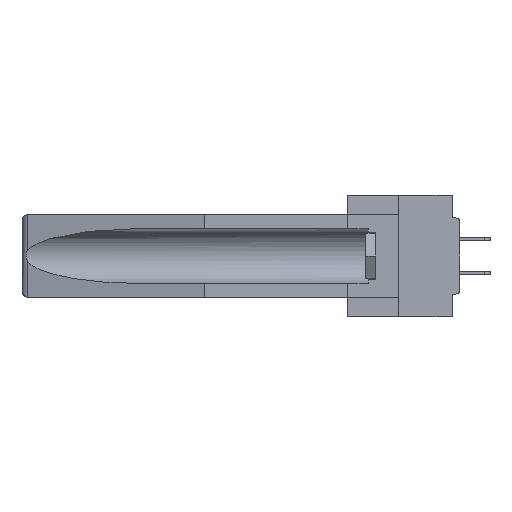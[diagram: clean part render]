
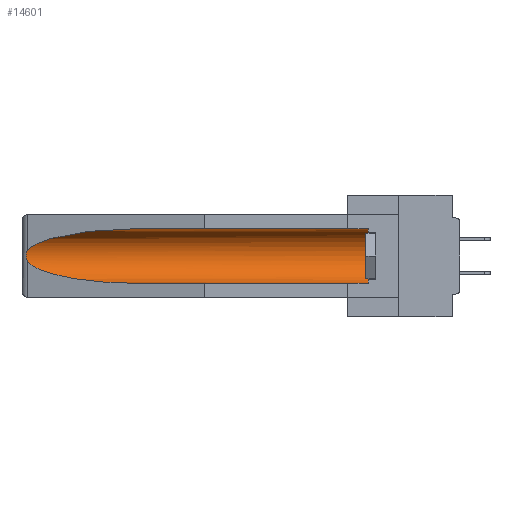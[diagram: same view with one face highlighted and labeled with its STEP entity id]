
A CAD part, left-side view. The second image highlights one B-rep face of the part: STEP entity #14601.
In plain terms, the highlighted cylindrical face has radius 2.857 mm (diameter 5.715 mm), a partial arc.
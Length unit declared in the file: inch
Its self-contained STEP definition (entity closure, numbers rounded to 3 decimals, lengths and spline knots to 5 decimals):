
#1794 = VERTEX_POINT ( 'NONE', #40493 ) ;
#1892 = AXIS2_PLACEMENT_3D ( 'NONE', #23911, #33760, #8006 ) ;
#2705 = ORIENTED_EDGE ( 'NONE', *, *, #22028, .F. ) ;
#3053 = CARTESIAN_POINT ( 'NONE',  ( 0.26537, 1.52718, -0.19328 ) ) ;
#3457 = EDGE_CURVE ( 'NONE', #14114, #29089, #15020, .T. ) ;
#5572 = CIRCLE ( 'NONE', #14593, 0.1125 ) ;
#5815 = CARTESIAN_POINT ( 'NONE',  ( 0.26537, 1.52718, -0.14972 ) ) ;
#6622 = DIRECTION ( 'NONE',  ( 0., 0., 1. ) ) ;
#7109 = ORIENTED_EDGE ( 'NONE', *, *, #8045, .T. ) ;
#7463 = EDGE_CURVE ( 'NONE', #29089, #35936, #31909, .T. ) ;
#7673 = EDGE_LOOP ( 'NONE', ( #7109, #12267, #18610, #2705, #37293, #23484 ) ) ;
#8006 = DIRECTION ( 'NONE',  ( 0., 0., 1. ) ) ;
#8045 = EDGE_CURVE ( 'NONE', #20190, #14114, #27569, .T. ) ;
#8701 = VERTEX_POINT ( 'NONE', #28786 ) ;
#8956 = CARTESIAN_POINT ( 'NONE',  ( 0.26654, 1.53092, -0.15636 ) ) ;
#10433 = FACE_OUTER_BOUND ( 'NONE', #7673, .T. ) ;
#10940 = CYLINDRICAL_SURFACE ( 'NONE', #1892, 0.1125 ) ;
#12159 = CARTESIAN_POINT ( 'NONE',  ( 0.26655, 1.53094, -0.18657 ) ) ;
#12267 = ORIENTED_EDGE ( 'NONE', *, *, #3457, .T. ) ;
#12301 = CARTESIAN_POINT ( 'NONE',  ( 0.2675, 1.53308, -0.16763 ) ) ;
#13319 = CARTESIAN_POINT ( 'NONE',  ( 0.155, 1.07973, -0.284 ) ) ;
#14114 = VERTEX_POINT ( 'NONE', #29840 ) ;
#14593 = AXIS2_PLACEMENT_3D ( 'NONE', #15925, #38287, #6622 ) ;
#14601 = ADVANCED_FACE ( 'NONE', ( #10433 ), #10940, .F. ) ;
#15020 = B_SPLINE_CURVE_WITH_KNOTS ( 'NONE', 3,
 ( #5815, #31403, #8956, #31123, #12301, #15354, #31261, #12159, #21824, #3053 ),
 .UNSPECIFIED., .F., .F.,
 ( 4, 2, 2, 2, 4 ),
 ( 0., 0.00029, 0.00058, 0.00087, 0.00117 ),
 .UNSPECIFIED. ) ;
#15200 = EDGE_CURVE ( 'NONE', #1794, #20190, #32361, .T. ) ;
#15354 = CARTESIAN_POINT ( 'NONE',  ( 0.2675, 1.53308, -0.17534 ) ) ;
#15822 = CARTESIAN_POINT ( 'NONE',  ( 0.155, 1.07973, -0.284 ) ) ;
#15885 = CARTESIAN_POINT ( 'NONE',  ( 0.155, 1.07973, -0.059 ) ) ;
#15925 = CARTESIAN_POINT ( 'NONE',  ( 0.155, 0.126, -0.1715 ) ) ;
#17012 = CARTESIAN_POINT ( 'NONE',  ( 0.26537, 1.52718, -0.14972 ) ) ;
#17506 = CARTESIAN_POINT ( 'NONE',  ( 0.26537, 1.52718, -0.19328 ) ) ;
#17642 = DIRECTION ( 'NONE',  ( 0., 1., 0. ) ) ;
#18610 = ORIENTED_EDGE ( 'NONE', *, *, #7463, .T. ) ;
#20097 = CARTESIAN_POINT ( 'NONE',  ( 0.21114, 1.30732, -0.059 ) ) ;
#20190 = VERTEX_POINT ( 'NONE', #15885 ) ;
#21824 = CARTESIAN_POINT ( 'NONE',  ( 0.26597, 1.5296, -0.19026 ) ) ;
#22028 = EDGE_CURVE ( 'NONE', #8701, #35936, #37632, .T. ) ;
#23181 = CARTESIAN_POINT ( 'NONE',  ( 0.155, 1.07973, -0.059 ) ) ;
#23484 = ORIENTED_EDGE ( 'NONE', *, *, #15200, .T. ) ;
#23568 = CARTESIAN_POINT ( 'NONE',  ( 0.25451, 1.48313, -0.09465 ) ) ;
#23911 = CARTESIAN_POINT ( 'NONE',  ( 0.155, -0.30754, -0.1715 ) ) ;
#24830 = EDGE_CURVE ( 'NONE', #8701, #1794, #5572, .T. ) ;
#25882 = CARTESIAN_POINT ( 'NONE',  ( 0.21114, 1.30732, -0.284 ) ) ;
#27569 =( BOUNDED_CURVE ( )  B_SPLINE_CURVE ( 3, ( #23181, #20097, #23568, #17012 ),
 .UNSPECIFIED., .F., .F. ) 
 B_SPLINE_CURVE_WITH_KNOTS ( ( 4, 4 ),
 ( 4.71239, 6.08839 ),
 .UNSPECIFIED. ) 
 CURVE ( )  GEOMETRIC_REPRESENTATION_ITEM ( )  RATIONAL_B_SPLINE_CURVE ( ( 1., 0.848, 0.848, 1. ) ) 
 REPRESENTATION_ITEM ( '' )  );
#28786 = CARTESIAN_POINT ( 'NONE',  ( 0.155, 0.126, -0.284 ) ) ;
#28879 = VECTOR ( 'NONE', #17642, 39.37008 ) ;
#29089 = VERTEX_POINT ( 'NONE', #37279 ) ;
#29840 = CARTESIAN_POINT ( 'NONE',  ( 0.26537, 1.52718, -0.14972 ) ) ;
#31123 = CARTESIAN_POINT ( 'NONE',  ( 0.2673, 1.5327, -0.16383 ) ) ;
#31261 = CARTESIAN_POINT ( 'NONE',  ( 0.2673, 1.53269, -0.17917 ) ) ;
#31403 = CARTESIAN_POINT ( 'NONE',  ( 0.26597, 1.52961, -0.15275 ) ) ;
#31909 =( BOUNDED_CURVE ( )  B_SPLINE_CURVE ( 3, ( #17506, #36694, #25882, #15822 ),
 .UNSPECIFIED., .F., .F. ) 
 B_SPLINE_CURVE_WITH_KNOTS ( ( 4, 4 ),
 ( 0.1948, 1.5708 ),
 .UNSPECIFIED. ) 
 CURVE ( )  GEOMETRIC_REPRESENTATION_ITEM ( )  RATIONAL_B_SPLINE_CURVE ( ( 1., 0.848, 0.848, 1. ) ) 
 REPRESENTATION_ITEM ( '' )  );
#32361 = LINE ( 'NONE', #33808, #28879 ) ;
#33760 = DIRECTION ( 'NONE',  ( 0., 1., 0. ) ) ;
#33808 = CARTESIAN_POINT ( 'NONE',  ( 0.155, -0.30754, -0.059 ) ) ;
#35936 = VERTEX_POINT ( 'NONE', #13319 ) ;
#36621 = VECTOR ( 'NONE', #37964, 39.37008 ) ;
#36694 = CARTESIAN_POINT ( 'NONE',  ( 0.25451, 1.48313, -0.24835 ) ) ;
#37279 = CARTESIAN_POINT ( 'NONE',  ( 0.26537, 1.52718, -0.19328 ) ) ;
#37293 = ORIENTED_EDGE ( 'NONE', *, *, #24830, .T. ) ;
#37632 = LINE ( 'NONE', #38108, #36621 ) ;
#37964 = DIRECTION ( 'NONE',  ( 0., 1., 0. ) ) ;
#38108 = CARTESIAN_POINT ( 'NONE',  ( 0.155, -0.30754, -0.284 ) ) ;
#38287 = DIRECTION ( 'NONE',  ( 0., -1., 0. ) ) ;
#40493 = CARTESIAN_POINT ( 'NONE',  ( 0.155, 0.126, -0.059 ) ) ;
